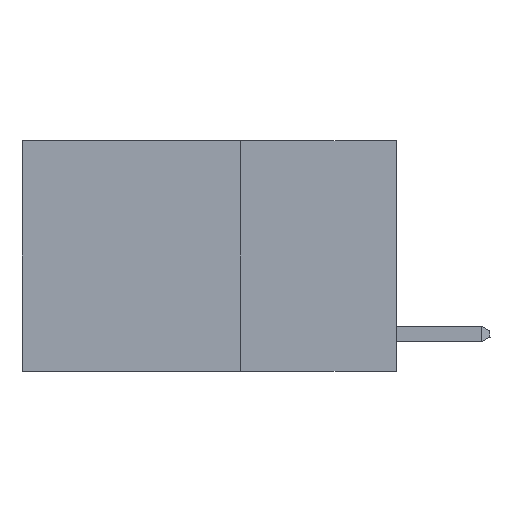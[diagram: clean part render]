
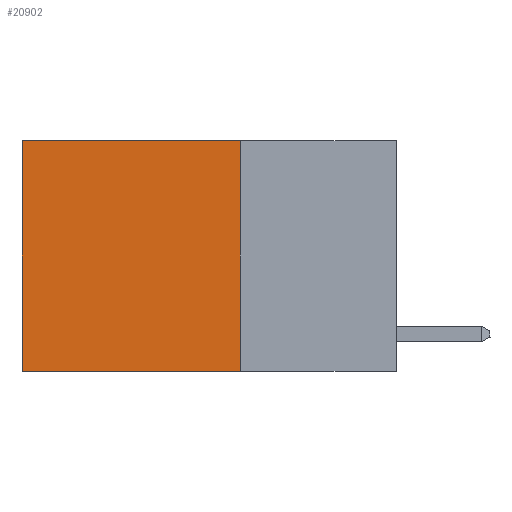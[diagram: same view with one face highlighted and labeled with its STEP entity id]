
A CAD part, left-side view. The second image highlights one B-rep face of the part: STEP entity #20902.
In plain terms, the highlighted planar face has unit normal (-1, 0, 0).
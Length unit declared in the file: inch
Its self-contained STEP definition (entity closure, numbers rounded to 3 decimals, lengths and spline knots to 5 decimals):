
#216 = LINE ( 'NONE', #20289, #8469 ) ;
#440 = EDGE_LOOP ( 'NONE', ( #16848, #2057, #10549, #19698 ) ) ;
#931 = PLANE ( 'NONE',  #2715 ) ;
#2057 = ORIENTED_EDGE ( 'NONE', *, *, #20111, .F. ) ;
#2715 = AXIS2_PLACEMENT_3D ( 'NONE', #9682, #2718, #14965 ) ;
#2718 = DIRECTION ( 'NONE',  ( 1., 0., 0. ) ) ;
#2739 = EDGE_CURVE ( 'NONE', #20920, #9077, #14810, .T. ) ;
#6644 = CARTESIAN_POINT ( 'NONE',  ( 0.2625, 0.25, 0. ) ) ;
#7233 = VECTOR ( 'NONE', #12657, 39.37008 ) ;
#8113 = FACE_OUTER_BOUND ( 'NONE', #440, .T. ) ;
#8469 = VECTOR ( 'NONE', #16851, 39.37008 ) ;
#8494 = DIRECTION ( 'NONE',  ( 0., 0., -1. ) ) ;
#9026 = VERTEX_POINT ( 'NONE', #10947 ) ;
#9077 = VERTEX_POINT ( 'NONE', #11102 ) ;
#9682 = CARTESIAN_POINT ( 'NONE',  ( 0.2625, 0.25, 0. ) ) ;
#9765 = CARTESIAN_POINT ( 'NONE',  ( 0.2625, 0.25, 0. ) ) ;
#10156 = VECTOR ( 'NONE', #8494, 39.37008 ) ;
#10549 = ORIENTED_EDGE ( 'NONE', *, *, #2739, .F. ) ;
#10947 = CARTESIAN_POINT ( 'NONE',  ( 0.2625, 0.6, -0.37 ) ) ;
#11082 = DIRECTION ( 'NONE',  ( 0., 1., 0. ) ) ;
#11102 = CARTESIAN_POINT ( 'NONE',  ( 0.2625, 0.25, -0.37 ) ) ;
#12657 = DIRECTION ( 'NONE',  ( 0., 0., -1. ) ) ;
#12860 = CARTESIAN_POINT ( 'NONE',  ( 0.2625, 0.25, -0.37 ) ) ;
#14450 = VECTOR ( 'NONE', #11082, 39.37008 ) ;
#14810 = LINE ( 'NONE', #6644, #10156 ) ;
#14965 = DIRECTION ( 'NONE',  ( 0., 0., -1. ) ) ;
#15260 = EDGE_CURVE ( 'NONE', #19943, #9026, #21205, .T. ) ;
#16848 = ORIENTED_EDGE ( 'NONE', *, *, #15260, .T. ) ;
#16851 = DIRECTION ( 'NONE',  ( 0., 1., 0. ) ) ;
#18475 = EDGE_CURVE ( 'NONE', #20920, #19943, #216, .T. ) ;
#19553 = CARTESIAN_POINT ( 'NONE',  ( 0.2625, 0.6, 0. ) ) ;
#19680 = LINE ( 'NONE', #12860, #14450 ) ;
#19698 = ORIENTED_EDGE ( 'NONE', *, *, #18475, .T. ) ;
#19943 = VERTEX_POINT ( 'NONE', #19553 ) ;
#20111 = EDGE_CURVE ( 'NONE', #9077, #9026, #19680, .T. ) ;
#20289 = CARTESIAN_POINT ( 'NONE',  ( 0.2625, 0.25, 0. ) ) ;
#20902 = ADVANCED_FACE ( 'NONE', ( #8113 ), #931, .F. ) ;
#20920 = VERTEX_POINT ( 'NONE', #9765 ) ;
#21205 = LINE ( 'NONE', #21371, #7233 ) ;
#21371 = CARTESIAN_POINT ( 'NONE',  ( 0.2625, 0.6, 0. ) ) ;
